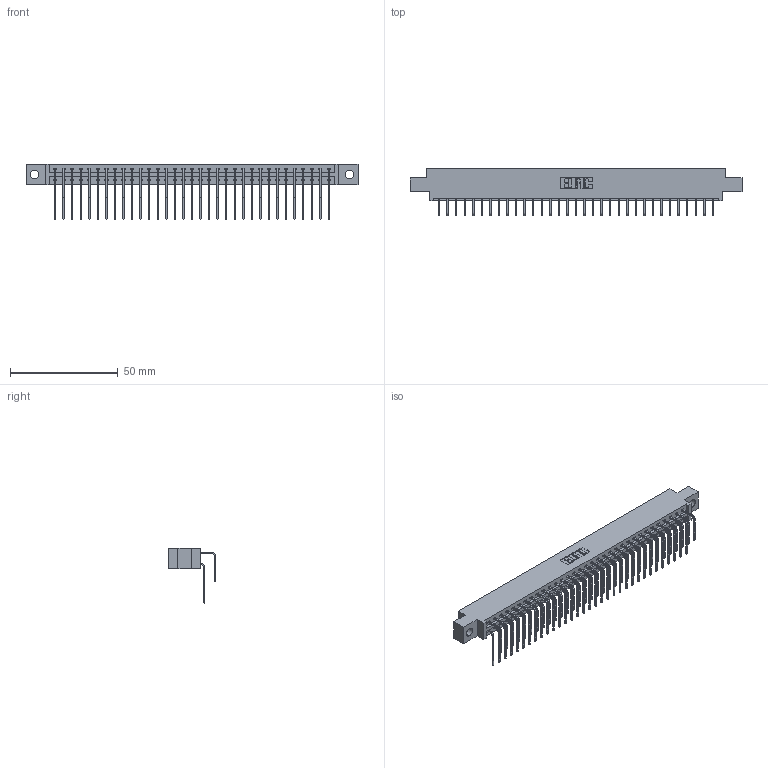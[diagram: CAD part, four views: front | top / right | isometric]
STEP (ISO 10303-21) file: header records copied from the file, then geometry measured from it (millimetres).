
FILE_DESCRIPTION (( 'STEP AP203' ), '1' );
FILE_NAME ('337-066-558-804.STEP', '2019-10-12T01:25:03', ( '' ), ( '' ), 'SwSTEP 2.0', 'SolidWorks 2016', '' );
FILE_SCHEMA (( 'CONFIG_CONTROL_DESIGN' ));
Length unit declared in the file: inch
Products named in the file (4): 345-292-001_558 559 Tail - 1; 337 Part_0.170 Offset - 0.156 Dia-TH; 345-292-001_558 Tail - 2; 337-066-558-804
Assembly tree (67 placements, depth 2):
  337-066-558-804
    337 Part_0.170 Offset - 0.156 Dia-TH
    345-292-001_558 559 Tail - 1  x33
    345-292-001_558 Tail - 2  x33
Bounding box: 153.77 x 22.17 x 25.53 mm (x, y, z)
Volume: 16261.2 mm3; surface area: 20112.9 mm2
Topology: 67 solids, 67 shells, 3814 faces, 11345 edges, 7474 vertices
Faces by surface type: plane 2714, cylinder 1100
Entity records: 28669 total; most frequent: CARTESIAN_POINT 4885, ORIENTED_EDGE 4770, DIRECTION 4153, EDGE_CURVE 2385, LINE 2217, VECTOR 2217, VERTEX_POINT 1586, AXIS2_PLACEMENT_3D 968
